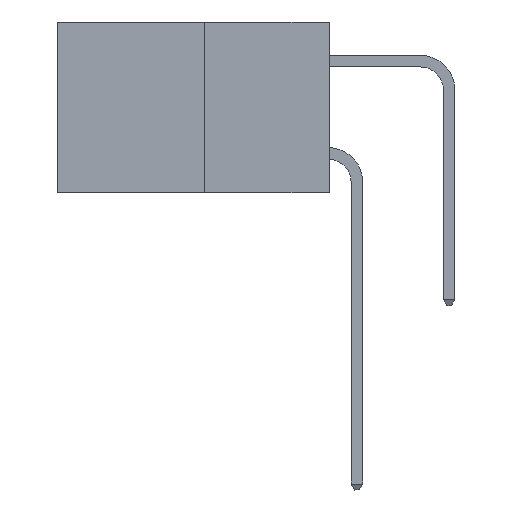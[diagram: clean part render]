
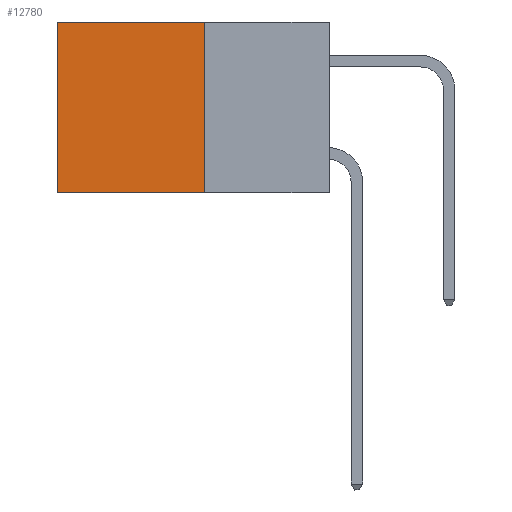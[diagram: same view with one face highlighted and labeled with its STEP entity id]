
A CAD part, left-side view. The second image highlights one B-rep face of the part: STEP entity #12780.
In plain terms, the highlighted planar face has unit normal (-1, 0, 0).
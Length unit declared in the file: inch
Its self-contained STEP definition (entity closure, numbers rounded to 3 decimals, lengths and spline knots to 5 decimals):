
#375 = LINE ( 'NONE', #21922, #14659 ) ;
#1206 = EDGE_CURVE ( 'NONE', #22163, #19443, #2178, .T. ) ;
#1473 = LINE ( 'NONE', #9310, #15672 ) ;
#1535 = CARTESIAN_POINT ( 'NONE',  ( 0.277, 0.59, 0. ) ) ;
#2178 = LINE ( 'NONE', #3303, #11932 ) ;
#2609 = VECTOR ( 'NONE', #7735, 39.37008 ) ;
#3116 = ORIENTED_EDGE ( 'NONE', *, *, #1206, .T. ) ;
#3303 = CARTESIAN_POINT ( 'NONE',  ( 0.277, 0.59, -0.37 ) ) ;
#3617 = ORIENTED_EDGE ( 'NONE', *, *, #5599, .F. ) ;
#3744 = CARTESIAN_POINT ( 'NONE',  ( 0.277, 0.27, 0. ) ) ;
#4006 = CARTESIAN_POINT ( 'NONE',  ( 0.277, 0.27, -0.37 ) ) ;
#4440 = FACE_OUTER_BOUND ( 'NONE', #9870, .T. ) ;
#5599 = EDGE_CURVE ( 'NONE', #17179, #19443, #17968, .T. ) ;
#5797 = ORIENTED_EDGE ( 'NONE', *, *, #15104, .F. ) ;
#6033 = PLANE ( 'NONE',  #8387 ) ;
#7735 = DIRECTION ( 'NONE',  ( 0., 1., 0. ) ) ;
#7964 = DIRECTION ( 'NONE',  ( 1., 0., 0. ) ) ;
#8387 = AXIS2_PLACEMENT_3D ( 'NONE', #4006, #7964, #21232 ) ;
#9298 = DIRECTION ( 'NONE',  ( 0., 0., -1. ) ) ;
#9310 = CARTESIAN_POINT ( 'NONE',  ( 0.277, 0.27, 0. ) ) ;
#9711 = ORIENTED_EDGE ( 'NONE', *, *, #18834, .T. ) ;
#9870 = EDGE_LOOP ( 'NONE', ( #3116, #3617, #5797, #9711 ) ) ;
#11932 = VECTOR ( 'NONE', #9298, 39.37008 ) ;
#12571 = DIRECTION ( 'NONE',  ( 0., 0., -1. ) ) ;
#12780 = ADVANCED_FACE ( 'NONE', ( #4440 ), #6033, .F. ) ;
#13540 = CARTESIAN_POINT ( 'NONE',  ( 0.277, 0.27, -0.37 ) ) ;
#14659 = VECTOR ( 'NONE', #12571, 39.37008 ) ;
#15071 = DIRECTION ( 'NONE',  ( 0., 1., 0. ) ) ;
#15104 = EDGE_CURVE ( 'NONE', #19506, #17179, #375, .T. ) ;
#15672 = VECTOR ( 'NONE', #15071, 39.37008 ) ;
#17179 = VERTEX_POINT ( 'NONE', #20023 ) ;
#17968 = LINE ( 'NONE', #13540, #2609 ) ;
#18834 = EDGE_CURVE ( 'NONE', #19506, #22163, #1473, .T. ) ;
#19443 = VERTEX_POINT ( 'NONE', #20744 ) ;
#19506 = VERTEX_POINT ( 'NONE', #3744 ) ;
#20023 = CARTESIAN_POINT ( 'NONE',  ( 0.277, 0.27, -0.37 ) ) ;
#20744 = CARTESIAN_POINT ( 'NONE',  ( 0.277, 0.59, -0.37 ) ) ;
#21232 = DIRECTION ( 'NONE',  ( 0., 0., -1. ) ) ;
#21922 = CARTESIAN_POINT ( 'NONE',  ( 0.277, 0.27, -0.37 ) ) ;
#22163 = VERTEX_POINT ( 'NONE', #1535 ) ;
